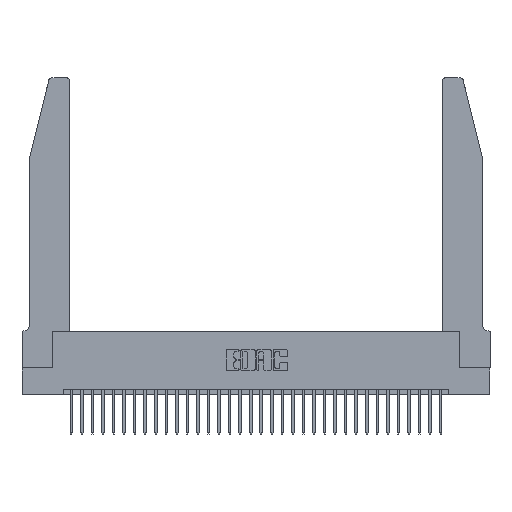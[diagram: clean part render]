
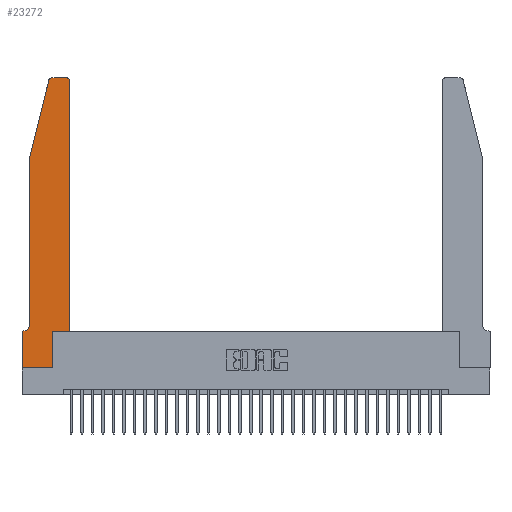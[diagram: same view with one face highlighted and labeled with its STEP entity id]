
A CAD part, top view. The second image highlights one B-rep face of the part: STEP entity #23272.
In plain terms, the highlighted planar face has unit normal (0, 0, 1).
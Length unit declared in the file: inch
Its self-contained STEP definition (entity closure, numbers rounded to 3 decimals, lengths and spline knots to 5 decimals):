
#1183 = EDGE_CURVE ( 'NONE', #16534, #10337, #27880, .T. ) ;
#1544 = EDGE_CURVE ( 'NONE', #20329, #24702, #2770, .T. ) ;
#2241 = EDGE_CURVE ( 'NONE', #25643, #12179, #4830, .T. ) ;
#2770 = CIRCLE ( 'NONE', #11064, 0.07 ) ;
#3149 = CARTESIAN_POINT ( 'NONE',  ( 0.2865, 0.35, 0.37 ) ) ;
#3767 = VECTOR ( 'NONE', #13349, 39.37008 ) ;
#4142 = VERTEX_POINT ( 'NONE', #7777 ) ;
#4168 = VERTEX_POINT ( 'NONE', #21998 ) ;
#4414 = EDGE_CURVE ( 'NONE', #4142, #20329, #8340, .T. ) ;
#4830 = LINE ( 'NONE', #10313, #8944 ) ;
#5928 = CARTESIAN_POINT ( 'NONE',  ( 0.0755, 2., 0.37 ) ) ;
#6399 = DIRECTION ( 'NONE',  ( -1., 0., 0. ) ) ;
#6423 = CARTESIAN_POINT ( 'NONE',  ( 0.0755, 0.35, 0.37 ) ) ;
#6520 = CARTESIAN_POINT ( 'NONE',  ( 0.0755, 2., 0.37 ) ) ;
#6583 = DIRECTION ( 'NONE',  ( 0., 0., 1. ) ) ;
#6885 = VECTOR ( 'NONE', #17463, 39.37008 ) ;
#7129 = AXIS2_PLACEMENT_3D ( 'NONE', #19362, #6583, #24981 ) ;
#7544 = LINE ( 'NONE', #3149, #3767 ) ;
#7743 = CARTESIAN_POINT ( 'NONE',  ( 0.4505, 0.35, 0.37 ) ) ;
#7777 = CARTESIAN_POINT ( 'NONE',  ( 0.0755, 2., 0.37 ) ) ;
#8340 = LINE ( 'NONE', #5928, #20245 ) ;
#8602 = CARTESIAN_POINT ( 'NONE',  ( 0.284, 2.75, 0.37 ) ) ;
#8944 = VECTOR ( 'NONE', #18792, 39.37008 ) ;
#9206 = CARTESIAN_POINT ( 'NONE',  ( 0.4505, 0.35, 0.37 ) ) ;
#9410 = CARTESIAN_POINT ( 'NONE',  ( 0.2605, 2.75, 0.37 ) ) ;
#9519 = CARTESIAN_POINT ( 'NONE',  ( 0.25487, 2.72718, 0.37 ) ) ;
#10313 = CARTESIAN_POINT ( 'NONE',  ( 0., 0., 0.37 ) ) ;
#10337 = VERTEX_POINT ( 'NONE', #19203 ) ;
#11064 = AXIS2_PLACEMENT_3D ( 'NONE', #17389, #12163, #22646 ) ;
#11144 = ORIENTED_EDGE ( 'NONE', *, *, #1544, .T. ) ;
#12163 = DIRECTION ( 'NONE',  ( 0., 0., -1. ) ) ;
#12172 = ORIENTED_EDGE ( 'NONE', *, *, #29246, .T. ) ;
#12179 = VERTEX_POINT ( 'NONE', #33055 ) ;
#12493 = VERTEX_POINT ( 'NONE', #21617 ) ;
#12733 = CIRCLE ( 'NONE', #7129, 0.03 ) ;
#13349 = DIRECTION ( 'NONE',  ( 0., 1., 0. ) ) ;
#13706 = ORIENTED_EDGE ( 'NONE', *, *, #29668, .T. ) ;
#13731 = EDGE_CURVE ( 'NONE', #12179, #12493, #7544, .T. ) ;
#14234 = DIRECTION ( 'NONE',  ( -1., 0., 0. ) ) ;
#14510 = VECTOR ( 'NONE', #25334, 39.37008 ) ;
#15109 = CARTESIAN_POINT ( 'NONE',  ( 0., 0., 0.37 ) ) ;
#15256 = EDGE_CURVE ( 'NONE', #10337, #18489, #25108, .T. ) ;
#15496 = LINE ( 'NONE', #15109, #6885 ) ;
#15529 = DIRECTION ( 'NONE',  ( 0., 0., 1. ) ) ;
#15742 = VECTOR ( 'NONE', #6399, 39.37008 ) ;
#16109 = ORIENTED_EDGE ( 'NONE', *, *, #29781, .T. ) ;
#16534 = VERTEX_POINT ( 'NONE', #9206 ) ;
#16669 = AXIS2_PLACEMENT_3D ( 'NONE', #31181, #15529, #28221 ) ;
#16928 = CARTESIAN_POINT ( 'NONE',  ( 0.0755, 0.42, 0.37 ) ) ;
#17114 = EDGE_CURVE ( 'NONE', #24702, #4168, #25805, .T. ) ;
#17389 = CARTESIAN_POINT ( 'NONE',  ( 0.0055, 0.42, 0.37 ) ) ;
#17463 = DIRECTION ( 'NONE',  ( 0., -1., 0. ) ) ;
#17586 = ORIENTED_EDGE ( 'NONE', *, *, #19484, .T. ) ;
#18160 = EDGE_LOOP ( 'NONE', ( #13706, #30765, #16109, #19654, #11144, #28908, #17586, #33743, #24431, #12172, #18963, #32117 ) ) ;
#18489 = VERTEX_POINT ( 'NONE', #19705 ) ;
#18792 = DIRECTION ( 'NONE',  ( 1., 0., 0. ) ) ;
#18963 = ORIENTED_EDGE ( 'NONE', *, *, #1183, .T. ) ;
#19137 = CARTESIAN_POINT ( 'NONE',  ( 0., 0., 0.37 ) ) ;
#19203 = CARTESIAN_POINT ( 'NONE',  ( 0.4505, 2.72, 0.37 ) ) ;
#19362 = CARTESIAN_POINT ( 'NONE',  ( 0.284, 2.72, 0.37 ) ) ;
#19484 = EDGE_CURVE ( 'NONE', #4168, #25643, #15496, .T. ) ;
#19654 = ORIENTED_EDGE ( 'NONE', *, *, #4414, .T. ) ;
#19705 = CARTESIAN_POINT ( 'NONE',  ( 0.4205, 2.75, 0.37 ) ) ;
#20088 = VECTOR ( 'NONE', #14234, 39.37008 ) ;
#20204 = LINE ( 'NONE', #6520, #33257 ) ;
#20245 = VECTOR ( 'NONE', #24228, 39.37008 ) ;
#20329 = VERTEX_POINT ( 'NONE', #16928 ) ;
#20721 = DIRECTION ( 'NONE',  ( 1., 0., 0. ) ) ;
#21378 = LINE ( 'NONE', #33179, #14510 ) ;
#21617 = CARTESIAN_POINT ( 'NONE',  ( 0.2865, 0.35, 0.37 ) ) ;
#21998 = CARTESIAN_POINT ( 'NONE',  ( 0., 0.35, 0.37 ) ) ;
#22646 = DIRECTION ( 'NONE',  ( -1., 0., 0. ) ) ;
#23272 = ADVANCED_FACE ( 'NONE', ( #25581 ), #25866, .T. ) ;
#23362 = DIRECTION ( 'NONE',  ( 0., 1., 0. ) ) ;
#24228 = DIRECTION ( 'NONE',  ( 0., -1., 0. ) ) ;
#24431 = ORIENTED_EDGE ( 'NONE', *, *, #13731, .T. ) ;
#24702 = VERTEX_POINT ( 'NONE', #29049 ) ;
#24811 = DIRECTION ( 'NONE',  ( -0.239, -0.971, 0. ) ) ;
#24981 = DIRECTION ( 'NONE',  ( 1., 0., 0. ) ) ;
#25108 = CIRCLE ( 'NONE', #16669, 0.03 ) ;
#25197 = VERTEX_POINT ( 'NONE', #9519 ) ;
#25334 = DIRECTION ( 'NONE',  ( 1., 0., 0. ) ) ;
#25385 = VECTOR ( 'NONE', #23362, 39.37008 ) ;
#25581 = FACE_OUTER_BOUND ( 'NONE', #18160, .T. ) ;
#25643 = VERTEX_POINT ( 'NONE', #19137 ) ;
#25805 = LINE ( 'NONE', #6423, #20088 ) ;
#25866 = PLANE ( 'NONE',  #32558 ) ;
#26094 = DIRECTION ( 'NONE',  ( 0., 0., 1. ) ) ;
#27880 = LINE ( 'NONE', #7743, #25385 ) ;
#28221 = DIRECTION ( 'NONE',  ( 1., 0., 0. ) ) ;
#28518 = CARTESIAN_POINT ( 'NONE',  ( 0., 0.35, 0.37 ) ) ;
#28908 = ORIENTED_EDGE ( 'NONE', *, *, #17114, .T. ) ;
#29049 = CARTESIAN_POINT ( 'NONE',  ( 0.0055, 0.35, 0.37 ) ) ;
#29246 = EDGE_CURVE ( 'NONE', #12493, #16534, #21378, .T. ) ;
#29668 = EDGE_CURVE ( 'NONE', #18489, #30419, #31624, .T. ) ;
#29781 = EDGE_CURVE ( 'NONE', #25197, #4142, #20204, .T. ) ;
#30419 = VERTEX_POINT ( 'NONE', #8602 ) ;
#30765 = ORIENTED_EDGE ( 'NONE', *, *, #31706, .T. ) ;
#31181 = CARTESIAN_POINT ( 'NONE',  ( 0.4205, 2.72, 0.37 ) ) ;
#31624 = LINE ( 'NONE', #9410, #15742 ) ;
#31706 = EDGE_CURVE ( 'NONE', #30419, #25197, #12733, .T. ) ;
#32117 = ORIENTED_EDGE ( 'NONE', *, *, #15256, .T. ) ;
#32558 = AXIS2_PLACEMENT_3D ( 'NONE', #28518, #26094, #20721 ) ;
#33055 = CARTESIAN_POINT ( 'NONE',  ( 0.2865, 0., 0.37 ) ) ;
#33179 = CARTESIAN_POINT ( 'NONE',  ( 0.4505, 0.35, 0.37 ) ) ;
#33257 = VECTOR ( 'NONE', #24811, 39.37008 ) ;
#33743 = ORIENTED_EDGE ( 'NONE', *, *, #2241, .T. ) ;
